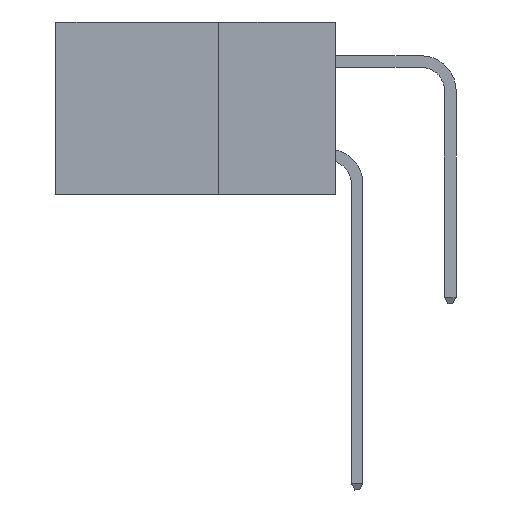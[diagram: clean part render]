
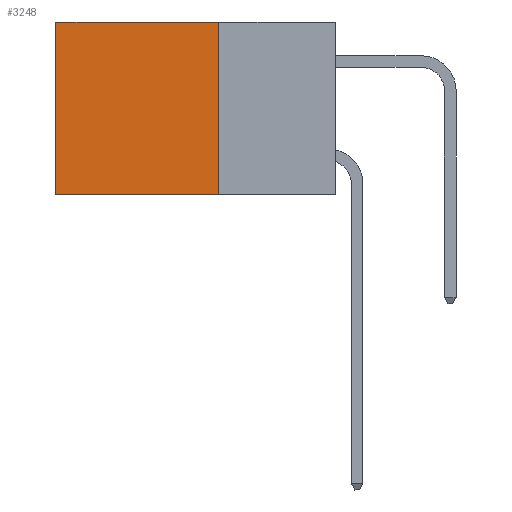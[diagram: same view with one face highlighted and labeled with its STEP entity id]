
A CAD part, left-side view. The second image highlights one B-rep face of the part: STEP entity #3248.
In plain terms, the highlighted planar face has unit normal (-1, 0, 0).
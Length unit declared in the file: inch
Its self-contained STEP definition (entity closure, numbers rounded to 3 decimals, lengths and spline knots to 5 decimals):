
#110 = LINE ( 'NONE', #2965, #12986 ) ;
#712 = ORIENTED_EDGE ( 'NONE', *, *, #2443, .T. ) ;
#2274 = AXIS2_PLACEMENT_3D ( 'NONE', #13594, #23290, #21522 ) ;
#2443 = EDGE_CURVE ( 'NONE', #15514, #9259, #110, .T. ) ;
#2965 = CARTESIAN_POINT ( 'NONE',  ( 0.2875, 0.6, 0. ) ) ;
#3034 = EDGE_CURVE ( 'NONE', #10550, #9259, #9381, .T. ) ;
#3085 = FACE_OUTER_BOUND ( 'NONE', #15285, .T. ) ;
#3248 = ADVANCED_FACE ( 'NONE', ( #3085 ), #6266, .F. ) ;
#4278 = VERTEX_POINT ( 'NONE', #13836 ) ;
#4322 = CARTESIAN_POINT ( 'NONE',  ( 0.2875, 0.6, -0.37 ) ) ;
#4425 = VECTOR ( 'NONE', #17001, 39.37008 ) ;
#5084 = CARTESIAN_POINT ( 'NONE',  ( 0.2875, 0.25, -0.37 ) ) ;
#6266 = PLANE ( 'NONE',  #2274 ) ;
#7436 = LINE ( 'NONE', #19181, #15292 ) ;
#8310 = LINE ( 'NONE', #19192, #4425 ) ;
#9259 = VERTEX_POINT ( 'NONE', #4322 ) ;
#9381 = LINE ( 'NONE', #20213, #17230 ) ;
#9948 = ORIENTED_EDGE ( 'NONE', *, *, #24714, .T. ) ;
#10550 = VERTEX_POINT ( 'NONE', #5084 ) ;
#11066 = ORIENTED_EDGE ( 'NONE', *, *, #3034, .F. ) ;
#12986 = VECTOR ( 'NONE', #21146, 39.37008 ) ;
#13594 = CARTESIAN_POINT ( 'NONE',  ( 0.2875, 0.25, 0. ) ) ;
#13836 = CARTESIAN_POINT ( 'NONE',  ( 0.2875, 0.25, 0. ) ) ;
#15285 = EDGE_LOOP ( 'NONE', ( #712, #11066, #23732, #9948 ) ) ;
#15292 = VECTOR ( 'NONE', #19755, 39.37008 ) ;
#15514 = VERTEX_POINT ( 'NONE', #18274 ) ;
#17001 = DIRECTION ( 'NONE',  ( 0., 1., 0. ) ) ;
#17014 = DIRECTION ( 'NONE',  ( 0., 1., 0. ) ) ;
#17230 = VECTOR ( 'NONE', #17014, 39.37008 ) ;
#18027 = EDGE_CURVE ( 'NONE', #4278, #10550, #7436, .T. ) ;
#18274 = CARTESIAN_POINT ( 'NONE',  ( 0.2875, 0.6, 0. ) ) ;
#19181 = CARTESIAN_POINT ( 'NONE',  ( 0.2875, 0.25, 0. ) ) ;
#19192 = CARTESIAN_POINT ( 'NONE',  ( 0.2875, 0.25, 0. ) ) ;
#19755 = DIRECTION ( 'NONE',  ( 0., 0., -1. ) ) ;
#20213 = CARTESIAN_POINT ( 'NONE',  ( 0.2875, 0.25, -0.37 ) ) ;
#21146 = DIRECTION ( 'NONE',  ( 0., 0., -1. ) ) ;
#21522 = DIRECTION ( 'NONE',  ( 0., 0., -1. ) ) ;
#23290 = DIRECTION ( 'NONE',  ( 1., 0., 0. ) ) ;
#23732 = ORIENTED_EDGE ( 'NONE', *, *, #18027, .F. ) ;
#24714 = EDGE_CURVE ( 'NONE', #4278, #15514, #8310, .T. ) ;
